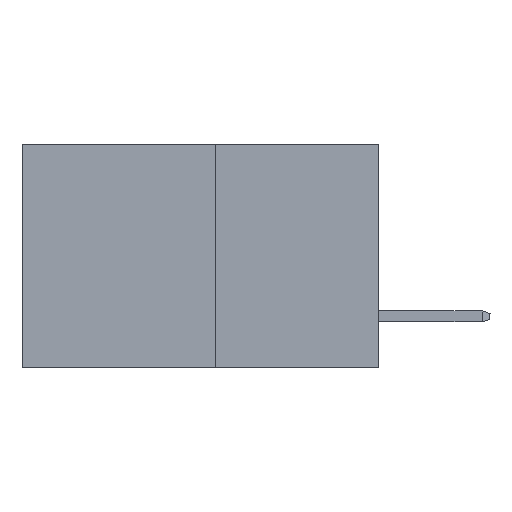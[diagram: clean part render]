
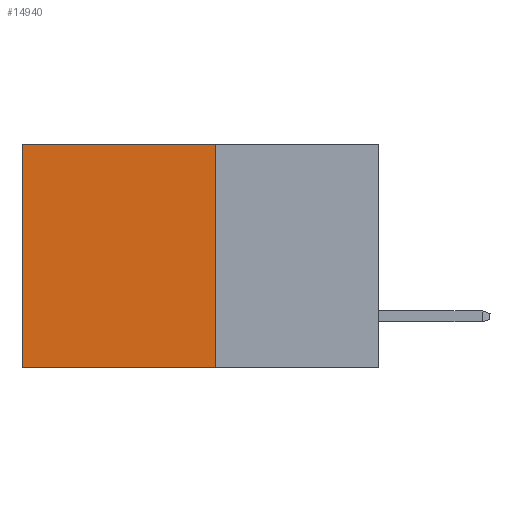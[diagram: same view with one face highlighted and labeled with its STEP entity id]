
A CAD part, left-side view. The second image highlights one B-rep face of the part: STEP entity #14940.
In plain terms, the highlighted planar face has unit normal (-1, 0, 0).
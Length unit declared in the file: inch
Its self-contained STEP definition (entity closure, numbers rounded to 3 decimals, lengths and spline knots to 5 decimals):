
#650 = VECTOR ( 'NONE', #8439, 39.37008 ) ;
#1097 = DIRECTION ( 'NONE',  ( 0., 0., -1. ) ) ;
#1112 = CARTESIAN_POINT ( 'NONE',  ( 0.277, 0.27, -0.37 ) ) ;
#1545 = ORIENTED_EDGE ( 'NONE', *, *, #11927, .T. ) ;
#2010 = EDGE_CURVE ( 'NONE', #13955, #10945, #4343, .T. ) ;
#2072 = CARTESIAN_POINT ( 'NONE',  ( 0.277, 0.27, 0. ) ) ;
#2520 = DIRECTION ( 'NONE',  ( 0., 0., -1. ) ) ;
#2803 = AXIS2_PLACEMENT_3D ( 'NONE', #9396, #10751, #2520 ) ;
#3641 = CARTESIAN_POINT ( 'NONE',  ( 0.277, 0.59, 0. ) ) ;
#4343 = LINE ( 'NONE', #8500, #650 ) ;
#4416 = VERTEX_POINT ( 'NONE', #10537 ) ;
#5280 = PLANE ( 'NONE',  #2803 ) ;
#6004 = VECTOR ( 'NONE', #1097, 39.37008 ) ;
#6972 = ORIENTED_EDGE ( 'NONE', *, *, #14012, .F. ) ;
#7272 = CARTESIAN_POINT ( 'NONE',  ( 0.277, 0.27, 0. ) ) ;
#8220 = EDGE_CURVE ( 'NONE', #13073, #4416, #17005, .T. ) ;
#8439 = DIRECTION ( 'NONE',  ( 0., 0., -1. ) ) ;
#8500 = CARTESIAN_POINT ( 'NONE',  ( 0.277, 0.59, -0.37 ) ) ;
#8724 = VECTOR ( 'NONE', #8960, 39.37008 ) ;
#8960 = DIRECTION ( 'NONE',  ( 0., 1., 0. ) ) ;
#9396 = CARTESIAN_POINT ( 'NONE',  ( 0.277, 0.27, -0.37 ) ) ;
#10537 = CARTESIAN_POINT ( 'NONE',  ( 0.277, 0.27, -0.37 ) ) ;
#10655 = CARTESIAN_POINT ( 'NONE',  ( 0.277, 0.27, -0.37 ) ) ;
#10751 = DIRECTION ( 'NONE',  ( 1., 0., 0. ) ) ;
#10945 = VERTEX_POINT ( 'NONE', #16935 ) ;
#11927 = EDGE_CURVE ( 'NONE', #13073, #13955, #15749, .T. ) ;
#13073 = VERTEX_POINT ( 'NONE', #7272 ) ;
#13955 = VERTEX_POINT ( 'NONE', #3641 ) ;
#14012 = EDGE_CURVE ( 'NONE', #4416, #10945, #15280, .T. ) ;
#14141 = ORIENTED_EDGE ( 'NONE', *, *, #2010, .T. ) ;
#14632 = DIRECTION ( 'NONE',  ( 0., 1., 0. ) ) ;
#14867 = VECTOR ( 'NONE', #14632, 39.37008 ) ;
#14940 = ADVANCED_FACE ( 'NONE', ( #16425 ), #5280, .F. ) ;
#15280 = LINE ( 'NONE', #10655, #14867 ) ;
#15749 = LINE ( 'NONE', #2072, #8724 ) ;
#16079 = EDGE_LOOP ( 'NONE', ( #14141, #6972, #16337, #1545 ) ) ;
#16337 = ORIENTED_EDGE ( 'NONE', *, *, #8220, .F. ) ;
#16425 = FACE_OUTER_BOUND ( 'NONE', #16079, .T. ) ;
#16935 = CARTESIAN_POINT ( 'NONE',  ( 0.277, 0.59, -0.37 ) ) ;
#17005 = LINE ( 'NONE', #1112, #6004 ) ;
